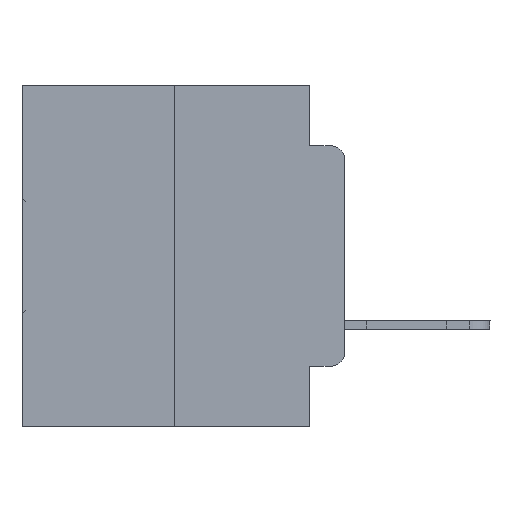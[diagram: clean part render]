
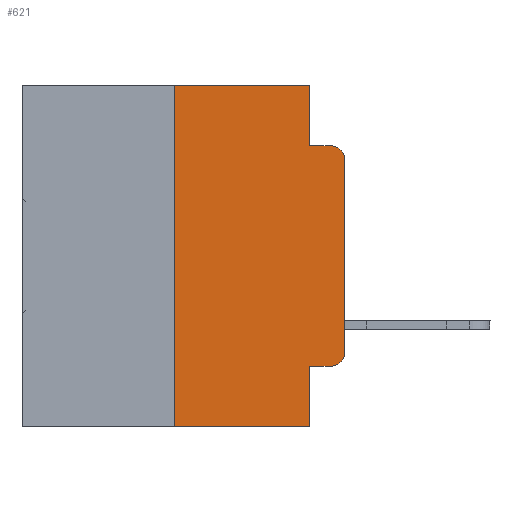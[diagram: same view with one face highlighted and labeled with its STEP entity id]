
A CAD part, left-side view. The second image highlights one B-rep face of the part: STEP entity #621.
In plain terms, the highlighted planar face has unit normal (-1, 0, 0).
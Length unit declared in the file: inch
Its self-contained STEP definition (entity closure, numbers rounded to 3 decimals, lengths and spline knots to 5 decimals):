
#1 = DIRECTION ( 'NONE',  ( 0., -1., 0. ) ) ;
#621 = ADVANCED_FACE ( 'NONE', ( #27177 ), #13379, .F. ) ;
#1112 = VERTEX_POINT ( 'NONE', #20616 ) ;
#1411 = DIRECTION ( 'NONE',  ( 0., 0., -1. ) ) ;
#1493 = AXIS2_PLACEMENT_3D ( 'NONE', #6688, #1863, #20647 ) ;
#1563 = VERTEX_POINT ( 'NONE', #10202 ) ;
#1643 = CARTESIAN_POINT ( 'NONE',  ( 0., 0.25, -0.5 ) ) ;
#1863 = DIRECTION ( 'NONE',  ( 1., 0., 0. ) ) ;
#2023 = VERTEX_POINT ( 'NONE', #29997 ) ;
#2514 = VERTEX_POINT ( 'NONE', #16437 ) ;
#2800 = LINE ( 'NONE', #4613, #24391 ) ;
#2842 = VERTEX_POINT ( 'NONE', #10117 ) ;
#3282 = DIRECTION ( 'NONE',  ( 0., -1., 0. ) ) ;
#3484 = EDGE_LOOP ( 'NONE', ( #13617, #11095, #24384, #10386, #25301, #10697, #22728, #21291, #6891, #7174 ) ) ;
#3787 = VERTEX_POINT ( 'NONE', #5105 ) ;
#3916 = LINE ( 'NONE', #20201, #20346 ) ;
#4029 = EDGE_CURVE ( 'NONE', #1563, #4651, #25451, .T. ) ;
#4613 = CARTESIAN_POINT ( 'NONE',  ( 0., 0.051, 0. ) ) ;
#4651 = VERTEX_POINT ( 'NONE', #26663 ) ;
#5105 = CARTESIAN_POINT ( 'NONE',  ( 0., 0.051, 0. ) ) ;
#5340 = DIRECTION ( 'NONE',  ( 0., -1., 0. ) ) ;
#5587 = EDGE_CURVE ( 'NONE', #18209, #2842, #27648, .T. ) ;
#5925 = DIRECTION ( 'NONE',  ( 0., -1., 0. ) ) ;
#6108 = EDGE_CURVE ( 'NONE', #13723, #2023, #29471, .T. ) ;
#6549 = VECTOR ( 'NONE', #1411, 39.37008 ) ;
#6688 = CARTESIAN_POINT ( 'NONE',  ( 0., 0.473, 0. ) ) ;
#6891 = ORIENTED_EDGE ( 'NONE', *, *, #26695, .T. ) ;
#7011 = DIRECTION ( 'NONE',  ( 0., 0., -1. ) ) ;
#7174 = ORIENTED_EDGE ( 'NONE', *, *, #5587, .T. ) ;
#7849 = VECTOR ( 'NONE', #1, 39.37008 ) ;
#8572 = VECTOR ( 'NONE', #5340, 39.37008 ) ;
#8600 = VECTOR ( 'NONE', #19453, 39.37008 ) ;
#9047 = EDGE_CURVE ( 'NONE', #2023, #3787, #3916, .T. ) ;
#10117 = CARTESIAN_POINT ( 'NONE',  ( 0., 0., -0.3915 ) ) ;
#10131 = CARTESIAN_POINT ( 'NONE',  ( 0., 0.02, -0.3915 ) ) ;
#10202 = CARTESIAN_POINT ( 'NONE',  ( 0., 0.051, -0.0885 ) ) ;
#10386 = ORIENTED_EDGE ( 'NONE', *, *, #11898, .F. ) ;
#10697 = ORIENTED_EDGE ( 'NONE', *, *, #6108, .F. ) ;
#10921 = CARTESIAN_POINT ( 'NONE',  ( 0., 0., 0. ) ) ;
#11095 = ORIENTED_EDGE ( 'NONE', *, *, #12572, .T. ) ;
#11151 = LINE ( 'NONE', #10921, #29801 ) ;
#11898 = EDGE_CURVE ( 'NONE', #3787, #1563, #25884, .T. ) ;
#12010 = DIRECTION ( 'NONE',  ( -1., 0., 0. ) ) ;
#12530 = DIRECTION ( 'NONE',  ( -1., 0., 0. ) ) ;
#12572 = EDGE_CURVE ( 'NONE', #1112, #4651, #29977, .T. ) ;
#12980 = VERTEX_POINT ( 'NONE', #29943 ) ;
#13379 = PLANE ( 'NONE',  #1493 ) ;
#13617 = ORIENTED_EDGE ( 'NONE', *, *, #16131, .T. ) ;
#13723 = VERTEX_POINT ( 'NONE', #1643 ) ;
#13841 = LINE ( 'NONE', #26082, #7849 ) ;
#16131 = EDGE_CURVE ( 'NONE', #2842, #1112, #11151, .T. ) ;
#16437 = CARTESIAN_POINT ( 'NONE',  ( 0., 0.051, -0.4115 ) ) ;
#17597 = CARTESIAN_POINT ( 'NONE',  ( 0., 0.051, -0.0885 ) ) ;
#17926 = LINE ( 'NONE', #22092, #8572 ) ;
#18209 = VERTEX_POINT ( 'NONE', #19221 ) ;
#19221 = CARTESIAN_POINT ( 'NONE',  ( 0., 0.02, -0.4115 ) ) ;
#19453 = DIRECTION ( 'NONE',  ( 0., 0., 1. ) ) ;
#20180 = EDGE_CURVE ( 'NONE', #13723, #12980, #17926, .T. ) ;
#20201 = CARTESIAN_POINT ( 'NONE',  ( 0., 0.473, 0. ) ) ;
#20346 = VECTOR ( 'NONE', #5925, 39.37008 ) ;
#20428 = CARTESIAN_POINT ( 'NONE',  ( 0., 0.051, 0. ) ) ;
#20616 = CARTESIAN_POINT ( 'NONE',  ( 0., 0., -0.1085 ) ) ;
#20647 = DIRECTION ( 'NONE',  ( 0., 0., -1. ) ) ;
#21212 = DIRECTION ( 'NONE',  ( 0., 0., 1. ) ) ;
#21291 = ORIENTED_EDGE ( 'NONE', *, *, #22596, .F. ) ;
#21740 = CARTESIAN_POINT ( 'NONE',  ( 0., 0.25, 0. ) ) ;
#22092 = CARTESIAN_POINT ( 'NONE',  ( 0., 0.473, -0.5 ) ) ;
#22596 = EDGE_CURVE ( 'NONE', #2514, #12980, #2800, .T. ) ;
#22728 = ORIENTED_EDGE ( 'NONE', *, *, #20180, .T. ) ;
#23538 = DIRECTION ( 'NONE',  ( 0., 0., -1. ) ) ;
#24384 = ORIENTED_EDGE ( 'NONE', *, *, #4029, .F. ) ;
#24391 = VECTOR ( 'NONE', #23538, 39.37008 ) ;
#25301 = ORIENTED_EDGE ( 'NONE', *, *, #9047, .F. ) ;
#25451 = LINE ( 'NONE', #17597, #29927 ) ;
#25884 = LINE ( 'NONE', #20428, #6549 ) ;
#25973 = AXIS2_PLACEMENT_3D ( 'NONE', #10131, #12530, #29184 ) ;
#26082 = CARTESIAN_POINT ( 'NONE',  ( 0., 0.051, -0.4115 ) ) ;
#26246 = CARTESIAN_POINT ( 'NONE',  ( 0., 0.02, -0.1085 ) ) ;
#26663 = CARTESIAN_POINT ( 'NONE',  ( 0., 0.02, -0.0885 ) ) ;
#26695 = EDGE_CURVE ( 'NONE', #2514, #18209, #13841, .T. ) ;
#27177 = FACE_OUTER_BOUND ( 'NONE', #3484, .T. ) ;
#27648 = CIRCLE ( 'NONE', #25973, 0.02 ) ;
#27731 = AXIS2_PLACEMENT_3D ( 'NONE', #26246, #12010, #7011 ) ;
#29184 = DIRECTION ( 'NONE',  ( 0., 0., -1. ) ) ;
#29471 = LINE ( 'NONE', #21740, #8600 ) ;
#29801 = VECTOR ( 'NONE', #21212, 39.37008 ) ;
#29927 = VECTOR ( 'NONE', #3282, 39.37008 ) ;
#29943 = CARTESIAN_POINT ( 'NONE',  ( 0., 0.051, -0.5 ) ) ;
#29977 = CIRCLE ( 'NONE', #27731, 0.02 ) ;
#29997 = CARTESIAN_POINT ( 'NONE',  ( 0., 0.25, 0. ) ) ;
